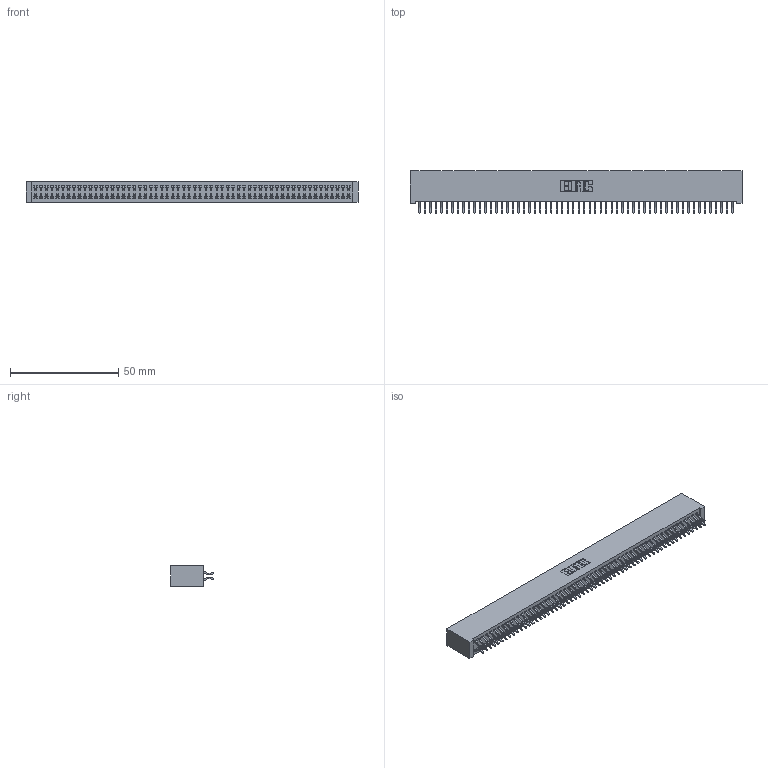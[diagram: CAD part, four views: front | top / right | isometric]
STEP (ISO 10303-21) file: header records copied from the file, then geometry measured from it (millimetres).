
FILE_DESCRIPTION (( 'STEP AP203' ), '1' );
FILE_NAME ('342-116-556-201.STEP', '2019-10-04T22:24:16', ( '' ), ( '' ), 'SwSTEP 2.0', 'SolidWorks 2016', '' );
FILE_SCHEMA (( 'CONFIG_CONTROL_DESIGN' ));
Length unit declared in the file: inch
Products named in the file (3): 342 Part_Lugless; 345-292-001_556 Tail; 342-116-556-201
Assembly tree (117 placements, depth 2):
  342-116-556-201
    342 Part_Lugless
    345-292-001_556 Tail  x116
Bounding box: 153.57 x 19.58 x 9.4 mm (x, y, z)
Volume: 14310.4 mm3; surface area: 24021.7 mm2
Topology: 117 solids, 117 shells, 6830 faces, 20343 edges, 13406 vertices
Faces by surface type: plane 4702, cylinder 2128
Entity records: 35055 total; most frequent: CARTESIAN_POINT 5802, ORIENTED_EDGE 5726, DIRECTION 4911, EDGE_CURVE 2863, VECTOR 2735, LINE 2735, VERTEX_POINT 1906, AXIS2_PLACEMENT_3D 1088
